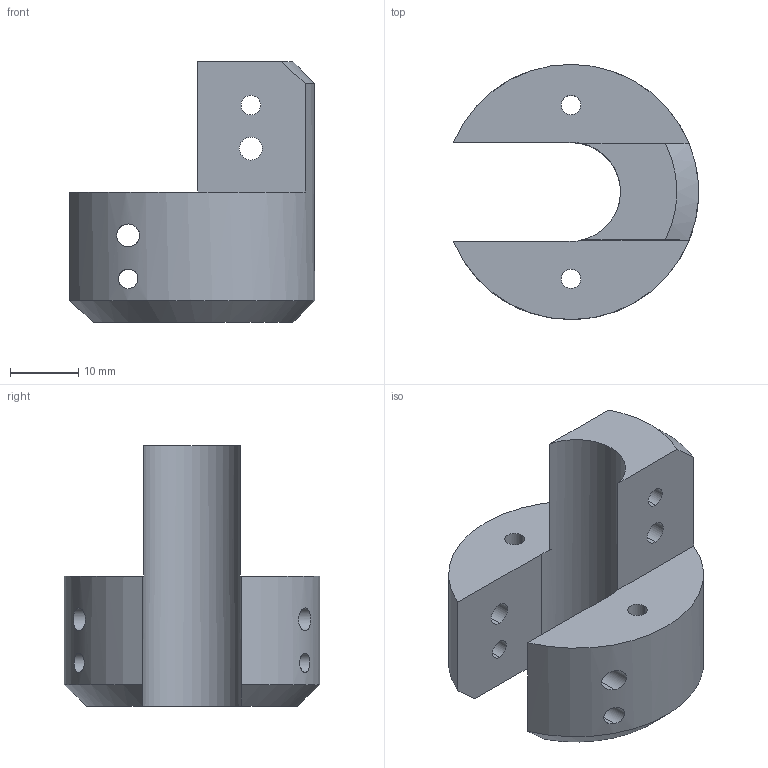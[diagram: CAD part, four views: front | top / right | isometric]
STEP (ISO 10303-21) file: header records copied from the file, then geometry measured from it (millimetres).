
FILE_DESCRIPTION (( 'STEP AP203' ), '1' );
FILE_NAME ('AF-RUGER1022NT-NTMCD-PRT-001-STEP.STEP', '2020-08-26T23:18:37', ( '' ), ( '' ), 'SwSTEP 2.0', 'SolidWorks 2018', '' );
FILE_SCHEMA (( 'CONFIG_CONTROL_DESIGN' ));
Length unit declared in the file: inch
Products named in the file (1): AF-RUGER1022NT-NTMCD-PRT-001-STEP
Bounding box: 35.88 x 37.34 x 38.1 mm (x, y, z)
Volume: 16316.9 mm3; surface area: 6388.9 mm2
Topology: 1 solids, 1 shells, 29 faces, 81 edges, 54 vertices
Faces by surface type: cylinder 18, plane 8, cone 3
Entity records: 1240 total; most frequent: CARTESIAN_POINT 367, DIRECTION 165, ORIENTED_EDGE 162, EDGE_CURVE 81, AXIS2_PLACEMENT_3D 66, VERTEX_POINT 54, EDGE_LOOP 45, CIRCLE 36
